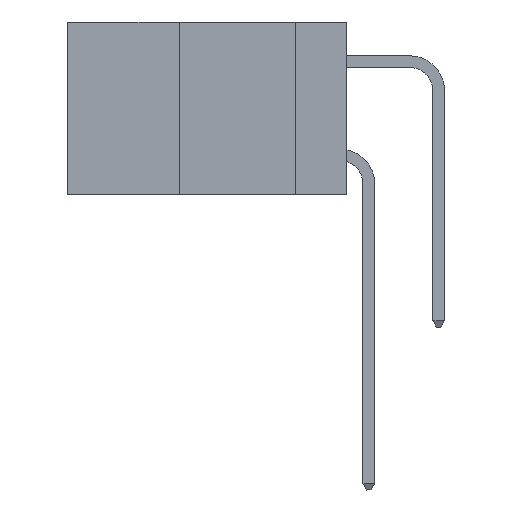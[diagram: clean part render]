
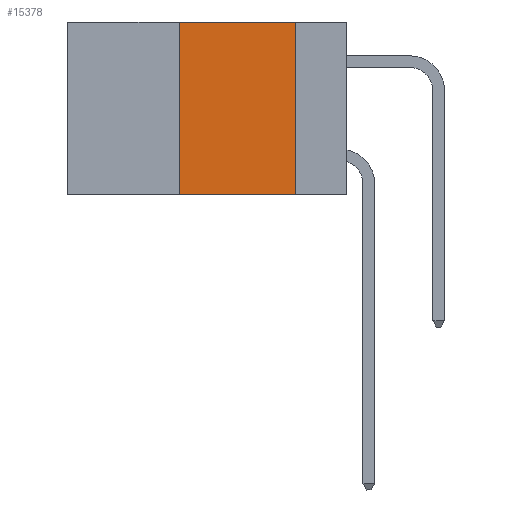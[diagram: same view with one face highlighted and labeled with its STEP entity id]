
A CAD part, left-side view. The second image highlights one B-rep face of the part: STEP entity #15378.
In plain terms, the highlighted planar face has unit normal (-1, 0, 0).
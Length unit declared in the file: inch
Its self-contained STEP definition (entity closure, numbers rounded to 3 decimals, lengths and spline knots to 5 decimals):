
#937 = VECTOR ( 'NONE', #21594, 39.37008 ) ;
#1841 = CARTESIAN_POINT ( 'NONE',  ( 0., 0.6, 0. ) ) ;
#2914 = DIRECTION ( 'NONE',  ( 0., 0., -1. ) ) ;
#3100 = EDGE_LOOP ( 'NONE', ( #3747, #4343, #5310, #5403 ) ) ;
#3747 = ORIENTED_EDGE ( 'NONE', *, *, #18404, .F. ) ;
#4343 = ORIENTED_EDGE ( 'NONE', *, *, #8895, .F. ) ;
#5310 = ORIENTED_EDGE ( 'NONE', *, *, #23949, .F. ) ;
#5403 = ORIENTED_EDGE ( 'NONE', *, *, #21452, .T. ) ;
#7137 = VERTEX_POINT ( 'NONE', #9018 ) ;
#7166 = FACE_OUTER_BOUND ( 'NONE', #3100, .T. ) ;
#7670 = DIRECTION ( 'NONE',  ( 0., 0., -1. ) ) ;
#8895 = EDGE_CURVE ( 'NONE', #22787, #22157, #11040, .T. ) ;
#9018 = CARTESIAN_POINT ( 'NONE',  ( 0., 0.36, -0.37 ) ) ;
#9458 = VERTEX_POINT ( 'NONE', #13576 ) ;
#10239 = CARTESIAN_POINT ( 'NONE',  ( 0., 0.6, -0.37 ) ) ;
#10883 = PLANE ( 'NONE',  #15534 ) ;
#10995 = CARTESIAN_POINT ( 'NONE',  ( 0., 0.36, 0. ) ) ;
#11040 = LINE ( 'NONE', #1841, #937 ) ;
#12259 = DIRECTION ( 'NONE',  ( 0., -1., 0. ) ) ;
#12674 = CARTESIAN_POINT ( 'NONE',  ( 0., 0.11, 0. ) ) ;
#12767 = CARTESIAN_POINT ( 'NONE',  ( 0., 0.36, 0. ) ) ;
#13533 = VECTOR ( 'NONE', #7670, 39.37008 ) ;
#13576 = CARTESIAN_POINT ( 'NONE',  ( 0., 0.11, -0.37 ) ) ;
#13595 = VECTOR ( 'NONE', #18621, 39.37008 ) ;
#14114 = LINE ( 'NONE', #24961, #13533 ) ;
#14789 = LINE ( 'NONE', #12767, #13595 ) ;
#14832 = DIRECTION ( 'NONE',  ( 1., 0., 0. ) ) ;
#15378 = ADVANCED_FACE ( 'NONE', ( #7166 ), #10883, .F. ) ;
#15534 = AXIS2_PLACEMENT_3D ( 'NONE', #24341, #14832, #2914 ) ;
#15812 = LINE ( 'NONE', #10239, #25319 ) ;
#18404 = EDGE_CURVE ( 'NONE', #22157, #9458, #14114, .T. ) ;
#18621 = DIRECTION ( 'NONE',  ( 0., 0., 1. ) ) ;
#21452 = EDGE_CURVE ( 'NONE', #7137, #9458, #15812, .T. ) ;
#21594 = DIRECTION ( 'NONE',  ( 0., -1., 0. ) ) ;
#22157 = VERTEX_POINT ( 'NONE', #12674 ) ;
#22787 = VERTEX_POINT ( 'NONE', #10995 ) ;
#23949 = EDGE_CURVE ( 'NONE', #7137, #22787, #14789, .T. ) ;
#24341 = CARTESIAN_POINT ( 'NONE',  ( 0., 0.6, 0. ) ) ;
#24961 = CARTESIAN_POINT ( 'NONE',  ( 0., 0.11, 0. ) ) ;
#25319 = VECTOR ( 'NONE', #12259, 39.37008 ) ;
